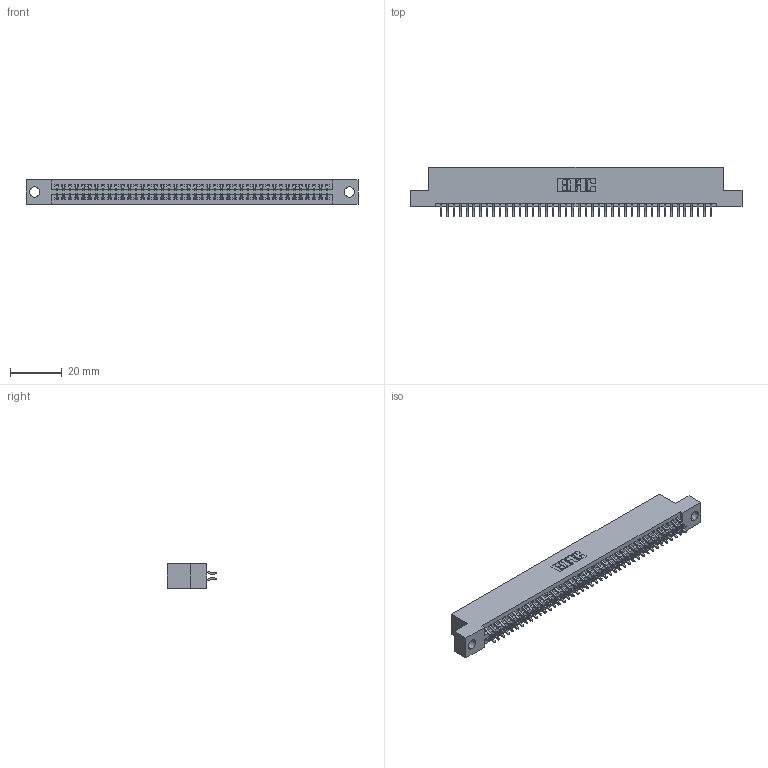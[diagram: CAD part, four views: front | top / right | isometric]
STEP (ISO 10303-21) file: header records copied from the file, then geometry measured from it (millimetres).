
FILE_DESCRIPTION (( 'STEP AP203' ), '1' );
FILE_NAME ('395-084-556-204.STEP', '2021-06-17T08:28:55', ( '' ), ( '' ), 'SwSTEP 2.0', 'SolidWorks 2020', '' );
FILE_SCHEMA (( 'CONFIG_CONTROL_DESIGN' ));
Length unit declared in the file: inch
Products named in the file (3): 395-084-556-204; 345 Part_Flush Mounting Lugs - 0.156 Dia-TI; 345-292-001_556 Tail
Assembly tree (85 placements, depth 2):
  395-084-556-204
    345 Part_Flush Mounting Lugs - 0.156 Dia-TI
    345-292-001_556 Tail  x84
Bounding box: 127.89 x 19.24 x 9.4 mm (x, y, z)
Volume: 12314 mm3; surface area: 17980.2 mm2
Topology: 85 solids, 85 shells, 4844 faces, 14405 edges, 9490 vertices
Faces by surface type: plane 3202, cylinder 1642
Entity records: 33593 total; most frequent: CARTESIAN_POINT 5650, ORIENTED_EDGE 5570, DIRECTION 4969, EDGE_CURVE 2785, LINE 2477, VECTOR 2477, VERTEX_POINT 1854, AXIS2_PLACEMENT_3D 1246
